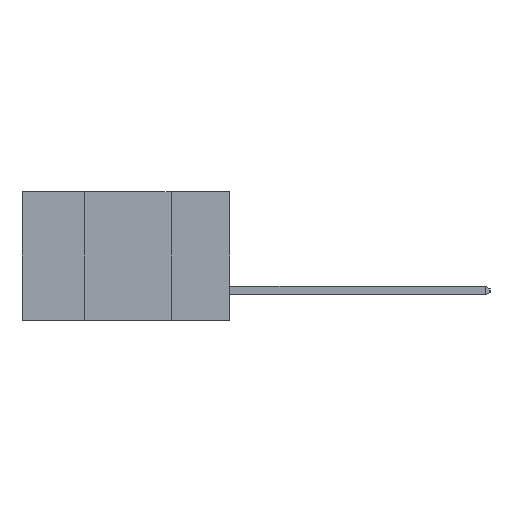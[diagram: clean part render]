
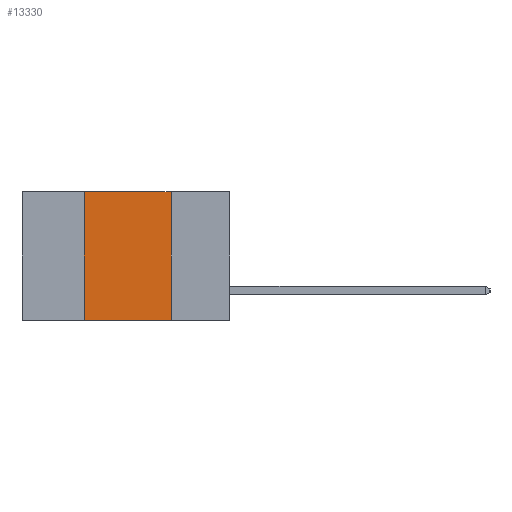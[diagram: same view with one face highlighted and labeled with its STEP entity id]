
A CAD part, left-side view. The second image highlights one B-rep face of the part: STEP entity #13330.
In plain terms, the highlighted planar face has unit normal (-1, 0, 0).
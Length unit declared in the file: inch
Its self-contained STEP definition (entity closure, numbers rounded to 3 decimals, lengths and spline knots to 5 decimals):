
#263 = LINE ( 'NONE', #19997, #26114 ) ;
#706 = LINE ( 'NONE', #18359, #19164 ) ;
#3351 = VERTEX_POINT ( 'NONE', #29224 ) ;
#4064 = EDGE_CURVE ( 'NONE', #3351, #8092, #28470, .T. ) ;
#6155 = CARTESIAN_POINT ( 'NONE',  ( 0., 0.6, 0. ) ) ;
#6538 = CARTESIAN_POINT ( 'NONE',  ( 0., 0.42, 0. ) ) ;
#8092 = VERTEX_POINT ( 'NONE', #30185 ) ;
#8498 = PLANE ( 'NONE',  #24565 ) ;
#8715 = DIRECTION ( 'NONE',  ( 0., 0., -1. ) ) ;
#9011 = EDGE_CURVE ( 'NONE', #29465, #19460, #16591, .T. ) ;
#11806 = DIRECTION ( 'NONE',  ( 0., -1., 0. ) ) ;
#12529 = DIRECTION ( 'NONE',  ( 0., 0., -1. ) ) ;
#13330 = ADVANCED_FACE ( 'NONE', ( #26065 ), #8498, .F. ) ;
#16326 = CARTESIAN_POINT ( 'NONE',  ( 0., 0.6, 0. ) ) ;
#16591 = LINE ( 'NONE', #16326, #28281 ) ;
#17543 = CARTESIAN_POINT ( 'NONE',  ( 0., 0.17, 0. ) ) ;
#17713 = ORIENTED_EDGE ( 'NONE', *, *, #9011, .F. ) ;
#18359 = CARTESIAN_POINT ( 'NONE',  ( 0., 0.42, 0. ) ) ;
#18833 = DIRECTION ( 'NONE',  ( 0., -1., 0. ) ) ;
#19164 = VECTOR ( 'NONE', #20863, 39.37008 ) ;
#19460 = VERTEX_POINT ( 'NONE', #17543 ) ;
#19997 = CARTESIAN_POINT ( 'NONE',  ( 0., 0.17, 0. ) ) ;
#20770 = EDGE_CURVE ( 'NONE', #19460, #8092, #263, .T. ) ;
#20863 = DIRECTION ( 'NONE',  ( 0., 0., 1. ) ) ;
#21086 = VECTOR ( 'NONE', #11806, 39.37008 ) ;
#21918 = CARTESIAN_POINT ( 'NONE',  ( 0., 0.6, -0.37 ) ) ;
#23753 = DIRECTION ( 'NONE',  ( 1., 0., 0. ) ) ;
#24565 = AXIS2_PLACEMENT_3D ( 'NONE', #6155, #23753, #8715 ) ;
#26065 = FACE_OUTER_BOUND ( 'NONE', #28022, .T. ) ;
#26114 = VECTOR ( 'NONE', #12529, 39.37008 ) ;
#26359 = ORIENTED_EDGE ( 'NONE', *, *, #20770, .F. ) ;
#27706 = ORIENTED_EDGE ( 'NONE', *, *, #30659, .F. ) ;
#28022 = EDGE_LOOP ( 'NONE', ( #26359, #17713, #27706, #31786 ) ) ;
#28281 = VECTOR ( 'NONE', #18833, 39.37008 ) ;
#28470 = LINE ( 'NONE', #21918, #21086 ) ;
#29224 = CARTESIAN_POINT ( 'NONE',  ( 0., 0.42, -0.37 ) ) ;
#29465 = VERTEX_POINT ( 'NONE', #6538 ) ;
#30185 = CARTESIAN_POINT ( 'NONE',  ( 0., 0.17, -0.37 ) ) ;
#30659 = EDGE_CURVE ( 'NONE', #3351, #29465, #706, .T. ) ;
#31786 = ORIENTED_EDGE ( 'NONE', *, *, #4064, .T. ) ;
